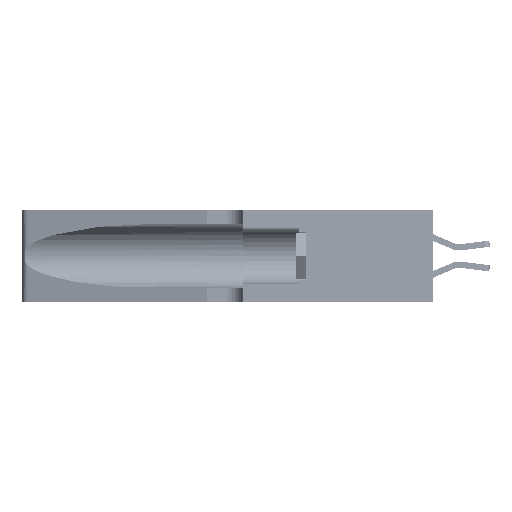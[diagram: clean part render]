
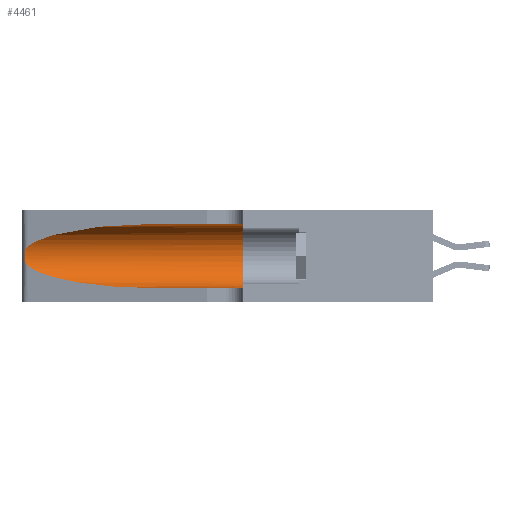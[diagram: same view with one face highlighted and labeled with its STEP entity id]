
A CAD part, left-side view. The second image highlights one B-rep face of the part: STEP entity #4461.
In plain terms, the highlighted cylindrical face has radius 3.308 mm (diameter 6.617 mm), a partial arc.
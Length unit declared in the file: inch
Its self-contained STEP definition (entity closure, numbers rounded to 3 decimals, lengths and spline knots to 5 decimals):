
#3676 = LINE ( 'NONE', #4549, #19093 ) ;
#4313 = CARTESIAN_POINT ( 'NONE',  ( 0.25487, 1.22718, 0.14631 ) ) ;
#4461 = ADVANCED_FACE ( 'NONE', ( #37786 ), #23944, .F. ) ;
#4531 = CARTESIAN_POINT ( 'NONE',  ( 0.2373, 1.15595, 0.08982 ) ) ;
#4549 = CARTESIAN_POINT ( 'NONE',  ( 0.1305, 1.61858, 0.05475 ) ) ;
#5133 = EDGE_CURVE ( 'NONE', #26871, #6987, #3676, .T. ) ;
#6461 = CARTESIAN_POINT ( 'NONE',  ( 0.25854, 1.2359, 0.20912 ) ) ;
#6987 = VERTEX_POINT ( 'NONE', #7407 ) ;
#7104 = EDGE_CURVE ( 'NONE', #16076, #40748, #40153, .T. ) ;
#7407 = CARTESIAN_POINT ( 'NONE',  ( 0.1305, 0.35, 0.05475 ) ) ;
#7604 = CARTESIAN_POINT ( 'NONE',  ( 0.1305, 0.72297, 0.05475 ) ) ;
#8054 = ORIENTED_EDGE ( 'NONE', *, *, #5133, .T. ) ;
#8719 = EDGE_LOOP ( 'NONE', ( #34363, #13655, #15520, #8054, #35665, #33805 ) ) ;
#11230 = EDGE_CURVE ( 'NONE', #33432, #26871, #42903, .T. ) ;
#13173 = CARTESIAN_POINT ( 'NONE',  ( 0.25856, 1.23593, 0.16098 ) ) ;
#13655 = ORIENTED_EDGE ( 'NONE', *, *, #26683, .T. ) ;
#14541 = CARTESIAN_POINT ( 'NONE',  ( 0.2373, 1.15595, 0.28018 ) ) ;
#14985 = CARTESIAN_POINT ( 'NONE',  ( 0.18966, 0.96281, 0.31525 ) ) ;
#15248 = CARTESIAN_POINT ( 'NONE',  ( 0.25487, 1.22718, 0.14631 ) ) ;
#15520 = ORIENTED_EDGE ( 'NONE', *, *, #11230, .T. ) ;
#15890 = DIRECTION ( 'NONE',  ( 0., 0., -1. ) ) ;
#16076 = VERTEX_POINT ( 'NONE', #16971 ) ;
#16715 = CARTESIAN_POINT ( 'NONE',  ( 0.26017, 1.23833, 0.17102 ) ) ;
#16971 = CARTESIAN_POINT ( 'NONE',  ( 0.1305, 0.72297, 0.31525 ) ) ;
#18207 = DIRECTION ( 'NONE',  ( 0., -1., 0. ) ) ;
#19093 = VECTOR ( 'NONE', #18207, 39.37008 ) ;
#19598 = VECTOR ( 'NONE', #43813, 39.37008 ) ;
#19715 = B_SPLINE_CURVE_WITH_KNOTS ( 'NONE', 3,
 ( #27238, #40188, #33516, #34986, #6461, #37055, #43652, #26659, #16715, #13173, #40473, #43936, #23710, #30524 ),
 .UNSPECIFIED., .F., .F.,
 ( 4, 2, 2, 2, 2, 2, 4 ),
 ( 0., 0.00027, 0.00053, 0.00107, 0.0016, 0.00187, 0.00214 ),
 .UNSPECIFIED. ) ;
#20283 = CARTESIAN_POINT ( 'NONE',  ( 0.1305, 0.35, 0.185 ) ) ;
#20584 = DIRECTION ( 'NONE',  ( 0., 1., 0. ) ) ;
#21204 = CARTESIAN_POINT ( 'NONE',  ( 0.1305, 0.72297, 0.31525 ) ) ;
#22799 = CARTESIAN_POINT ( 'NONE',  ( 0.18966, 0.96281, 0.05475 ) ) ;
#23155 = DIRECTION ( 'NONE',  ( 0., -1., 0. ) ) ;
#23240 = AXIS2_PLACEMENT_3D ( 'NONE', #20283, #20584, #26978 ) ;
#23710 = CARTESIAN_POINT ( 'NONE',  ( 0.25555, 1.22993, 0.14849 ) ) ;
#23944 = CYLINDRICAL_SURFACE ( 'NONE', #29471, 0.13025 ) ;
#24954 = LINE ( 'NONE', #43965, #19598 ) ;
#26659 = CARTESIAN_POINT ( 'NONE',  ( 0.26075, 1.23896, 0.178 ) ) ;
#26683 = EDGE_CURVE ( 'NONE', #40748, #33432, #19715, .T. ) ;
#26871 = VERTEX_POINT ( 'NONE', #7604 ) ;
#26978 = DIRECTION ( 'NONE',  ( 0., 0., 1. ) ) ;
#27238 = CARTESIAN_POINT ( 'NONE',  ( 0.25487, 1.22718, 0.22369 ) ) ;
#27551 = CIRCLE ( 'NONE', #23240, 0.13025 ) ;
#29471 = AXIS2_PLACEMENT_3D ( 'NONE', #36358, #23155, #15890 ) ;
#30524 = CARTESIAN_POINT ( 'NONE',  ( 0.25487, 1.22718, 0.14631 ) ) ;
#32600 = CARTESIAN_POINT ( 'NONE',  ( 0.1305, 0.35, 0.31525 ) ) ;
#33432 = VERTEX_POINT ( 'NONE', #4313 ) ;
#33516 = CARTESIAN_POINT ( 'NONE',  ( 0.25639, 1.23184, 0.21858 ) ) ;
#33805 = ORIENTED_EDGE ( 'NONE', *, *, #37613, .F. ) ;
#34363 = ORIENTED_EDGE ( 'NONE', *, *, #7104, .T. ) ;
#34986 = CARTESIAN_POINT ( 'NONE',  ( 0.25787, 1.23484, 0.2124 ) ) ;
#35665 = ORIENTED_EDGE ( 'NONE', *, *, #37583, .F. ) ;
#36358 = CARTESIAN_POINT ( 'NONE',  ( 0.1305, 1.61858, 0.185 ) ) ;
#36434 = CARTESIAN_POINT ( 'NONE',  ( 0.1305, 0.72297, 0.05475 ) ) ;
#37055 = CARTESIAN_POINT ( 'NONE',  ( 0.26018, 1.23835, 0.19895 ) ) ;
#37583 = EDGE_CURVE ( 'NONE', #38151, #6987, #27551, .T. ) ;
#37613 = EDGE_CURVE ( 'NONE', #16076, #38151, #24954, .T. ) ;
#37786 = FACE_OUTER_BOUND ( 'NONE', #8719, .T. ) ;
#38151 = VERTEX_POINT ( 'NONE', #32600 ) ;
#40153 =( BOUNDED_CURVE ( )  B_SPLINE_CURVE ( 3, ( #21204, #14985, #14541, #41402 ),
 .UNSPECIFIED., .F., .F. ) 
 B_SPLINE_CURVE_WITH_KNOTS ( ( 4, 4 ),
 ( 1.5708, 2.84003 ),
 .UNSPECIFIED. ) 
 CURVE ( )  GEOMETRIC_REPRESENTATION_ITEM ( )  RATIONAL_B_SPLINE_CURVE ( ( 1., 0.87, 0.87, 1. ) ) 
 REPRESENTATION_ITEM ( '' )  );
#40188 = CARTESIAN_POINT ( 'NONE',  ( 0.25555, 1.22994, 0.2215 ) ) ;
#40473 = CARTESIAN_POINT ( 'NONE',  ( 0.25789, 1.23486, 0.15765 ) ) ;
#40748 = VERTEX_POINT ( 'NONE', #43703 ) ;
#41402 = CARTESIAN_POINT ( 'NONE',  ( 0.25487, 1.22718, 0.22369 ) ) ;
#42903 =( BOUNDED_CURVE ( )  B_SPLINE_CURVE ( 3, ( #15248, #4531, #22799, #36434 ),
 .UNSPECIFIED., .F., .F. ) 
 B_SPLINE_CURVE_WITH_KNOTS ( ( 4, 4 ),
 ( 3.44316, 4.71239 ),
 .UNSPECIFIED. ) 
 CURVE ( )  GEOMETRIC_REPRESENTATION_ITEM ( )  RATIONAL_B_SPLINE_CURVE ( ( 1., 0.87, 0.87, 1. ) ) 
 REPRESENTATION_ITEM ( '' )  );
#43652 = CARTESIAN_POINT ( 'NONE',  ( 0.26075, 1.23896, 0.19203 ) ) ;
#43703 = CARTESIAN_POINT ( 'NONE',  ( 0.25487, 1.22718, 0.22369 ) ) ;
#43813 = DIRECTION ( 'NONE',  ( 0., -1., 0. ) ) ;
#43936 = CARTESIAN_POINT ( 'NONE',  ( 0.25639, 1.23186, 0.15144 ) ) ;
#43965 = CARTESIAN_POINT ( 'NONE',  ( 0.1305, 1.61858, 0.31525 ) ) ;
